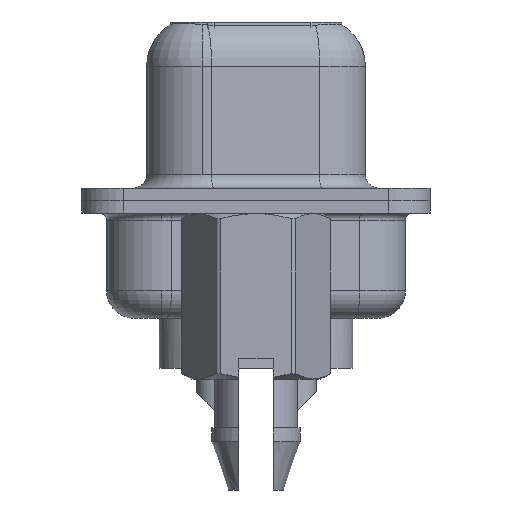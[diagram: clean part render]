
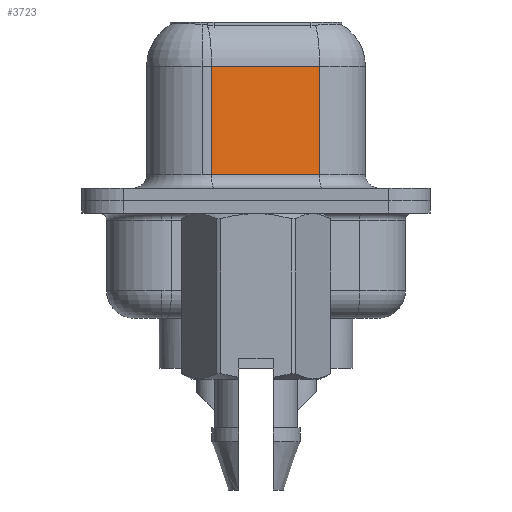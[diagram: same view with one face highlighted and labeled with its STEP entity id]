
A CAD part, left-side view. The second image highlights one B-rep face of the part: STEP entity #3723.
In plain terms, the highlighted planar face has unit normal (-0.985, -0.174, 0).
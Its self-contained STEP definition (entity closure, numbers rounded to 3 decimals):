
#191 = LINE ( 'NONE', #6447, #5090 ) ;
#404 = PLANE ( 'NONE',  #17680 ) ;
#1471 = VERTEX_POINT ( 'NONE', #10857 ) ;
#1742 = FACE_OUTER_BOUND ( 'NONE', #12261, .T. ) ;
#1829 = ORIENTED_EDGE ( 'NONE', *, *, #3776, .F. ) ;
#1939 = DIRECTION ( 'NONE',  ( -0.174, 0.985, 0. ) ) ;
#2330 = CARTESIAN_POINT ( 'NONE',  ( 4.375, 1.603, 6.6 ) ) ;
#2685 = DIRECTION ( 'NONE',  ( 0.174, -0.985, 0. ) ) ;
#3723 = ADVANCED_FACE ( 'NONE', ( #1742 ), #404, .F. ) ;
#3776 = EDGE_CURVE ( 'NONE', #12867, #15277, #191, .T. ) ;
#4035 = LINE ( 'NONE', #19538, #9435 ) ;
#5090 = VECTOR ( 'NONE', #12714, 1000. ) ;
#5265 = VECTOR ( 'NONE', #5611, 1000. ) ;
#5611 = DIRECTION ( 'NONE',  ( 0., 0., -1. ) ) ;
#6447 = CARTESIAN_POINT ( 'NONE',  ( 5.063, -2.297, 6.6 ) ) ;
#6657 = CARTESIAN_POINT ( 'NONE',  ( 5.063, -2.297, 6.6 ) ) ;
#7678 = CARTESIAN_POINT ( 'NONE',  ( 4.375, 1.603, 0.95 ) ) ;
#8001 = DIRECTION ( 'NONE',  ( 0.985, 0.174, 0. ) ) ;
#8031 = ORIENTED_EDGE ( 'NONE', *, *, #19853, .T. ) ;
#8183 = CARTESIAN_POINT ( 'NONE',  ( 5.063, -2.297, 4.85 ) ) ;
#9435 = VECTOR ( 'NONE', #2685, 1000. ) ;
#9731 = ORIENTED_EDGE ( 'NONE', *, *, #17763, .T. ) ;
#9745 = DIRECTION ( 'NONE',  ( -0.174, 0.985, 0. ) ) ;
#10857 = CARTESIAN_POINT ( 'NONE',  ( 4.375, 1.603, 4.85 ) ) ;
#10914 = VECTOR ( 'NONE', #1939, 1000. ) ;
#11967 = ORIENTED_EDGE ( 'NONE', *, *, #15316, .T. ) ;
#12261 = EDGE_LOOP ( 'NONE', ( #1829, #9731, #11967, #8031 ) ) ;
#12714 = DIRECTION ( 'NONE',  ( 0., 0., -1. ) ) ;
#12808 = CARTESIAN_POINT ( 'NONE',  ( 5.063, -2.297, 4.85 ) ) ;
#12867 = VERTEX_POINT ( 'NONE', #8183 ) ;
#13899 = VERTEX_POINT ( 'NONE', #7678 ) ;
#15277 = VERTEX_POINT ( 'NONE', #19668 ) ;
#15316 = EDGE_CURVE ( 'NONE', #1471, #13899, #16405, .T. ) ;
#16405 = LINE ( 'NONE', #2330, #5265 ) ;
#17602 = LINE ( 'NONE', #12808, #10914 ) ;
#17680 = AXIS2_PLACEMENT_3D ( 'NONE', #6657, #8001, #9745 ) ;
#17763 = EDGE_CURVE ( 'NONE', #12867, #1471, #17602, .T. ) ;
#19538 = CARTESIAN_POINT ( 'NONE',  ( 5.063, -2.297, 0.95 ) ) ;
#19668 = CARTESIAN_POINT ( 'NONE',  ( 5.063, -2.297, 0.95 ) ) ;
#19853 = EDGE_CURVE ( 'NONE', #13899, #15277, #4035, .T. ) ;
